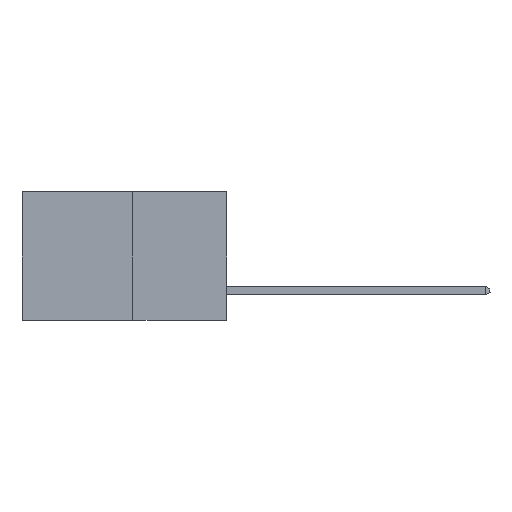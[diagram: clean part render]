
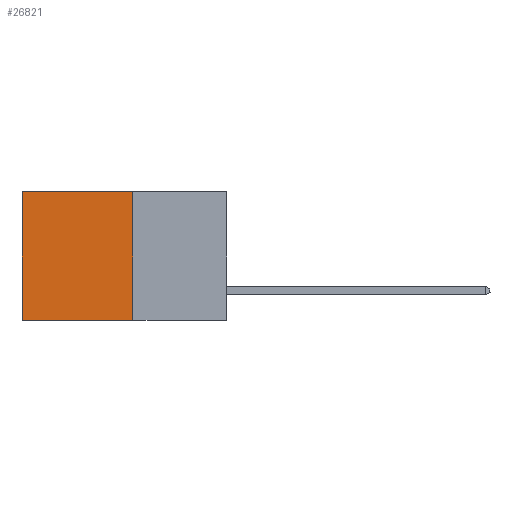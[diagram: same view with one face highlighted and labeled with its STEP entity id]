
A CAD part, left-side view. The second image highlights one B-rep face of the part: STEP entity #26821.
In plain terms, the highlighted planar face has unit normal (-1, 0, 0).
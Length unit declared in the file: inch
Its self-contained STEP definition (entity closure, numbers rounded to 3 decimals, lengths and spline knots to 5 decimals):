
#1443 = VECTOR ( 'NONE', #1633, 39.37008 ) ;
#1633 = DIRECTION ( 'NONE',  ( 0., 1., 0. ) ) ;
#1924 = CARTESIAN_POINT ( 'NONE',  ( 0.277, 0.27, 0. ) ) ;
#2215 = LINE ( 'NONE', #1924, #1443 ) ;
#4637 = LINE ( 'NONE', #8327, #23038 ) ;
#5710 = EDGE_CURVE ( 'NONE', #20680, #27867, #14948, .T. ) ;
#5893 = CARTESIAN_POINT ( 'NONE',  ( 0.277, 0.27, -0.37 ) ) ;
#6471 = AXIS2_PLACEMENT_3D ( 'NONE', #23384, #9543, #25758 ) ;
#7355 = VERTEX_POINT ( 'NONE', #16356 ) ;
#8184 = DIRECTION ( 'NONE',  ( 0., 0., -1. ) ) ;
#8327 = CARTESIAN_POINT ( 'NONE',  ( 0.277, 0.27, -0.37 ) ) ;
#8805 = VECTOR ( 'NONE', #27185, 39.37008 ) ;
#8849 = CARTESIAN_POINT ( 'NONE',  ( 0.277, 0.59, 0. ) ) ;
#9543 = DIRECTION ( 'NONE',  ( 1., 0., 0. ) ) ;
#10686 = CARTESIAN_POINT ( 'NONE',  ( 0.277, 0.59, -0.37 ) ) ;
#13391 = EDGE_CURVE ( 'NONE', #7355, #20680, #2215, .T. ) ;
#14266 = ORIENTED_EDGE ( 'NONE', *, *, #15189, .F. ) ;
#14948 = LINE ( 'NONE', #27532, #8805 ) ;
#15189 = EDGE_CURVE ( 'NONE', #18980, #27867, #4637, .T. ) ;
#16157 = FACE_OUTER_BOUND ( 'NONE', #18786, .T. ) ;
#16356 = CARTESIAN_POINT ( 'NONE',  ( 0.277, 0.27, 0. ) ) ;
#17285 = ORIENTED_EDGE ( 'NONE', *, *, #24346, .F. ) ;
#18786 = EDGE_LOOP ( 'NONE', ( #29499, #14266, #17285, #28599 ) ) ;
#18980 = VERTEX_POINT ( 'NONE', #27058 ) ;
#20680 = VERTEX_POINT ( 'NONE', #8849 ) ;
#21085 = PLANE ( 'NONE',  #6471 ) ;
#21247 = VECTOR ( 'NONE', #8184, 39.37008 ) ;
#23038 = VECTOR ( 'NONE', #29102, 39.37008 ) ;
#23384 = CARTESIAN_POINT ( 'NONE',  ( 0.277, 0.27, -0.37 ) ) ;
#23402 = LINE ( 'NONE', #5893, #21247 ) ;
#24346 = EDGE_CURVE ( 'NONE', #7355, #18980, #23402, .T. ) ;
#25758 = DIRECTION ( 'NONE',  ( 0., 0., -1. ) ) ;
#26821 = ADVANCED_FACE ( 'NONE', ( #16157 ), #21085, .F. ) ;
#27058 = CARTESIAN_POINT ( 'NONE',  ( 0.277, 0.27, -0.37 ) ) ;
#27185 = DIRECTION ( 'NONE',  ( 0., 0., -1. ) ) ;
#27532 = CARTESIAN_POINT ( 'NONE',  ( 0.277, 0.59, -0.37 ) ) ;
#27867 = VERTEX_POINT ( 'NONE', #10686 ) ;
#28599 = ORIENTED_EDGE ( 'NONE', *, *, #13391, .T. ) ;
#29102 = DIRECTION ( 'NONE',  ( 0., 1., 0. ) ) ;
#29499 = ORIENTED_EDGE ( 'NONE', *, *, #5710, .T. ) ;
